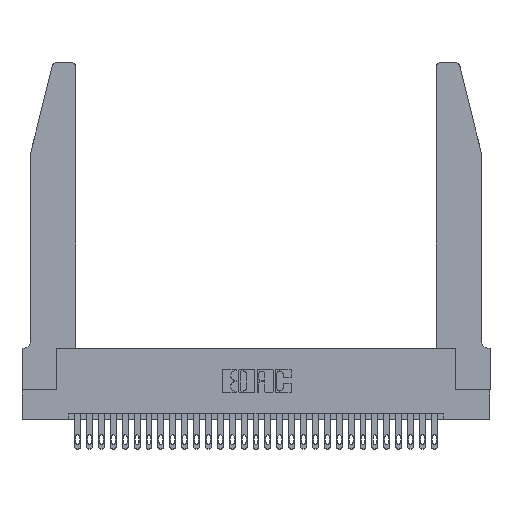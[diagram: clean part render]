
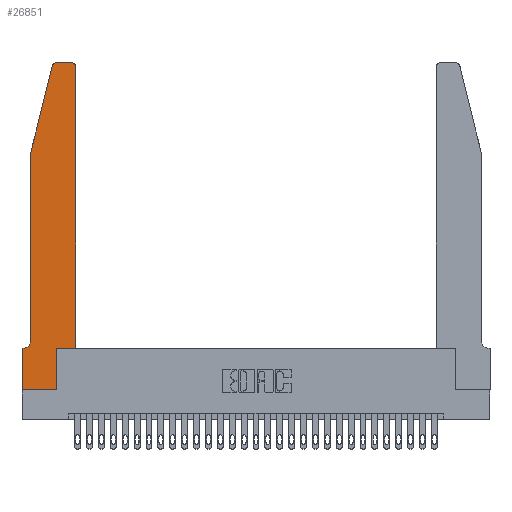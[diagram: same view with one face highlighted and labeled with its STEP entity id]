
A CAD part, top view. The second image highlights one B-rep face of the part: STEP entity #26851.
In plain terms, the highlighted planar face has unit normal (0, 0, 1).
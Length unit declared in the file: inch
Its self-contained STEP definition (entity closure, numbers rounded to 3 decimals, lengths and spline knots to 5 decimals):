
#55 = EDGE_LOOP ( 'NONE', ( #20638, #21233, #2461, #9378, #13034, #26149, #29962, #8993, #23192, #7778, #547, #5978 ) ) ;
#547 = ORIENTED_EDGE ( 'NONE', *, *, #8988, .T. ) ;
#890 = DIRECTION ( 'NONE',  ( 0., 0., -1. ) ) ;
#2461 = ORIENTED_EDGE ( 'NONE', *, *, #26212, .T. ) ;
#2495 = VERTEX_POINT ( 'NONE', #3772 ) ;
#2648 = EDGE_CURVE ( 'NONE', #6420, #4586, #22206, .T. ) ;
#3139 = EDGE_CURVE ( 'NONE', #4918, #6660, #22567, .T. ) ;
#3202 = VERTEX_POINT ( 'NONE', #15576 ) ;
#3772 = CARTESIAN_POINT ( 'NONE',  ( 0., 0.35, 0.37 ) ) ;
#3872 = CARTESIAN_POINT ( 'NONE',  ( 0.2865, 0.35, 0.37 ) ) ;
#4079 = CARTESIAN_POINT ( 'NONE',  ( 0.284, 2.72, 0.37 ) ) ;
#4387 = AXIS2_PLACEMENT_3D ( 'NONE', #13186, #890, #20121 ) ;
#4459 = DIRECTION ( 'NONE',  ( 0., 0., 1. ) ) ;
#4586 = VERTEX_POINT ( 'NONE', #20860 ) ;
#4728 = CARTESIAN_POINT ( 'NONE',  ( 0.0055, 0.35, 0.37 ) ) ;
#4876 = CARTESIAN_POINT ( 'NONE',  ( 0., 0., 0.37 ) ) ;
#4918 = VERTEX_POINT ( 'NONE', #8273 ) ;
#5294 = LINE ( 'NONE', #12146, #9111 ) ;
#5978 = ORIENTED_EDGE ( 'NONE', *, *, #3139, .T. ) ;
#6420 = VERTEX_POINT ( 'NONE', #8053 ) ;
#6660 = VERTEX_POINT ( 'NONE', #14092 ) ;
#7620 = VECTOR ( 'NONE', #12382, 39.37008 ) ;
#7778 = ORIENTED_EDGE ( 'NONE', *, *, #26307, .T. ) ;
#8053 = CARTESIAN_POINT ( 'NONE',  ( 0.284, 2.75, 0.37 ) ) ;
#8273 = CARTESIAN_POINT ( 'NONE',  ( 0.4505, 2.72, 0.37 ) ) ;
#8988 = EDGE_CURVE ( 'NONE', #16589, #4918, #9552, .T. ) ;
#8993 = ORIENTED_EDGE ( 'NONE', *, *, #27346, .T. ) ;
#9014 = VECTOR ( 'NONE', #30031, 39.37008 ) ;
#9034 = CARTESIAN_POINT ( 'NONE',  ( 0.2605, 2.75, 0.37 ) ) ;
#9111 = VECTOR ( 'NONE', #14536, 39.37008 ) ;
#9378 = ORIENTED_EDGE ( 'NONE', *, *, #15202, .T. ) ;
#9552 = LINE ( 'NONE', #19363, #26865 ) ;
#9648 = EDGE_CURVE ( 'NONE', #29858, #2495, #13192, .T. ) ;
#9816 = CARTESIAN_POINT ( 'NONE',  ( 0.4205, 2.72, 0.37 ) ) ;
#10076 = CARTESIAN_POINT ( 'NONE',  ( 0.0755, 2., 0.37 ) ) ;
#10170 = LINE ( 'NONE', #21201, #17939 ) ;
#10677 = EDGE_CURVE ( 'NONE', #26818, #29858, #21649, .T. ) ;
#11658 = FACE_OUTER_BOUND ( 'NONE', #55, .T. ) ;
#11786 = EDGE_CURVE ( 'NONE', #3202, #22988, #14208, .T. ) ;
#11931 = CARTESIAN_POINT ( 'NONE',  ( 0.4505, 0.35, 0.37 ) ) ;
#12033 = DIRECTION ( 'NONE',  ( 0., -1., 0. ) ) ;
#12146 = CARTESIAN_POINT ( 'NONE',  ( 0.4505, 0.35, 0.37 ) ) ;
#12382 = DIRECTION ( 'NONE',  ( -1., 0., 0. ) ) ;
#12836 = CARTESIAN_POINT ( 'NONE',  ( 0., 0., 0.37 ) ) ;
#12962 = AXIS2_PLACEMENT_3D ( 'NONE', #9816, #21894, #26704 ) ;
#13034 = ORIENTED_EDGE ( 'NONE', *, *, #10677, .T. ) ;
#13186 = CARTESIAN_POINT ( 'NONE',  ( 0.0055, 0.42, 0.37 ) ) ;
#13192 = LINE ( 'NONE', #24409, #7620 ) ;
#13290 = DIRECTION ( 'NONE',  ( 0., 1., 0. ) ) ;
#13591 = EDGE_CURVE ( 'NONE', #2495, #27182, #14821, .T. ) ;
#13813 = CARTESIAN_POINT ( 'NONE',  ( 0.0755, 0.42, 0.37 ) ) ;
#13913 = CARTESIAN_POINT ( 'NONE',  ( 0., 0.35, 0.37 ) ) ;
#14092 = CARTESIAN_POINT ( 'NONE',  ( 0.4205, 2.75, 0.37 ) ) ;
#14201 = VECTOR ( 'NONE', #25249, 39.37008 ) ;
#14208 = LINE ( 'NONE', #3872, #17923 ) ;
#14536 = DIRECTION ( 'NONE',  ( 1., 0., 0. ) ) ;
#14821 = LINE ( 'NONE', #4876, #20031 ) ;
#15202 = EDGE_CURVE ( 'NONE', #17144, #26818, #29062, .T. ) ;
#15576 = CARTESIAN_POINT ( 'NONE',  ( 0.2865, 0., 0.37 ) ) ;
#16582 = VECTOR ( 'NONE', #27032, 39.37008 ) ;
#16589 = VERTEX_POINT ( 'NONE', #11931 ) ;
#16682 = CARTESIAN_POINT ( 'NONE',  ( 0.2865, 0.35, 0.37 ) ) ;
#17144 = VERTEX_POINT ( 'NONE', #10076 ) ;
#17293 = EDGE_CURVE ( 'NONE', #6660, #6420, #26720, .T. ) ;
#17923 = VECTOR ( 'NONE', #13290, 39.37008 ) ;
#17939 = VECTOR ( 'NONE', #21302, 39.37008 ) ;
#18127 = CARTESIAN_POINT ( 'NONE',  ( 0., 0., 0.37 ) ) ;
#19363 = CARTESIAN_POINT ( 'NONE',  ( 0.4505, 0.35, 0.37 ) ) ;
#19854 = AXIS2_PLACEMENT_3D ( 'NONE', #13913, #4459, #21057 ) ;
#20031 = VECTOR ( 'NONE', #12033, 39.37008 ) ;
#20121 = DIRECTION ( 'NONE',  ( -1., 0., 0. ) ) ;
#20638 = ORIENTED_EDGE ( 'NONE', *, *, #17293, .T. ) ;
#20650 = DIRECTION ( 'NONE',  ( 0., 0., 1. ) ) ;
#20860 = CARTESIAN_POINT ( 'NONE',  ( 0.25487, 2.72718, 0.37 ) ) ;
#21057 = DIRECTION ( 'NONE',  ( 1., 0., 0. ) ) ;
#21201 = CARTESIAN_POINT ( 'NONE',  ( 0.0755, 2., 0.37 ) ) ;
#21233 = ORIENTED_EDGE ( 'NONE', *, *, #2648, .T. ) ;
#21302 = DIRECTION ( 'NONE',  ( -0.239, -0.971, 0. ) ) ;
#21649 = CIRCLE ( 'NONE', #4387, 0.07 ) ;
#21894 = DIRECTION ( 'NONE',  ( 0., 0., 1. ) ) ;
#22206 = CIRCLE ( 'NONE', #22478, 0.03 ) ;
#22478 = AXIS2_PLACEMENT_3D ( 'NONE', #4079, #20650, #23036 ) ;
#22567 = CIRCLE ( 'NONE', #12962, 0.03 ) ;
#22988 = VERTEX_POINT ( 'NONE', #16682 ) ;
#23036 = DIRECTION ( 'NONE',  ( 1., 0., 0. ) ) ;
#23192 = ORIENTED_EDGE ( 'NONE', *, *, #11786, .T. ) ;
#24409 = CARTESIAN_POINT ( 'NONE',  ( 0.0755, 0.35, 0.37 ) ) ;
#25249 = DIRECTION ( 'NONE',  ( 1., 0., 0. ) ) ;
#25380 = PLANE ( 'NONE',  #19854 ) ;
#26149 = ORIENTED_EDGE ( 'NONE', *, *, #9648, .T. ) ;
#26212 = EDGE_CURVE ( 'NONE', #4586, #17144, #10170, .T. ) ;
#26307 = EDGE_CURVE ( 'NONE', #22988, #16589, #5294, .T. ) ;
#26704 = DIRECTION ( 'NONE',  ( 1., 0., 0. ) ) ;
#26720 = LINE ( 'NONE', #9034, #9014 ) ;
#26818 = VERTEX_POINT ( 'NONE', #13813 ) ;
#26851 = ADVANCED_FACE ( 'NONE', ( #11658 ), #25380, .T. ) ;
#26865 = VECTOR ( 'NONE', #28906, 39.37008 ) ;
#27032 = DIRECTION ( 'NONE',  ( 0., -1., 0. ) ) ;
#27182 = VERTEX_POINT ( 'NONE', #12836 ) ;
#27346 = EDGE_CURVE ( 'NONE', #27182, #3202, #30393, .T. ) ;
#28906 = DIRECTION ( 'NONE',  ( 0., 1., 0. ) ) ;
#29062 = LINE ( 'NONE', #29272, #16582 ) ;
#29272 = CARTESIAN_POINT ( 'NONE',  ( 0.0755, 2., 0.37 ) ) ;
#29858 = VERTEX_POINT ( 'NONE', #4728 ) ;
#29962 = ORIENTED_EDGE ( 'NONE', *, *, #13591, .T. ) ;
#30031 = DIRECTION ( 'NONE',  ( -1., 0., 0. ) ) ;
#30393 = LINE ( 'NONE', #18127, #14201 ) ;
